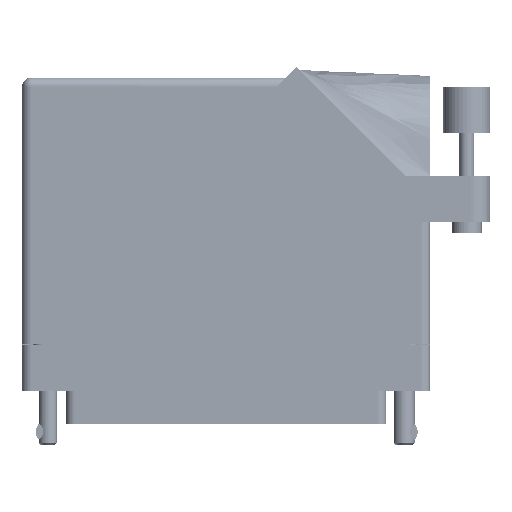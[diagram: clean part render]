
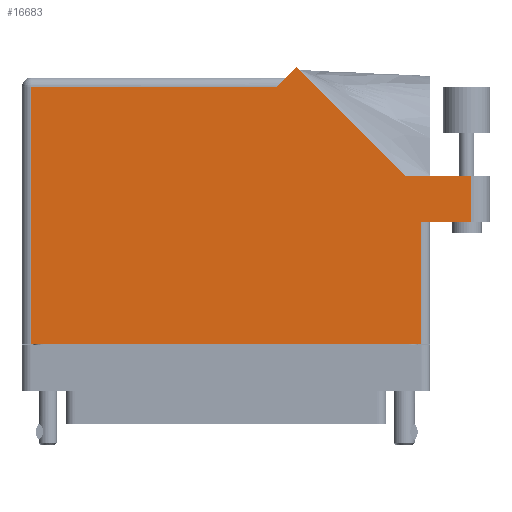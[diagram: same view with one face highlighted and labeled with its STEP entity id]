
A CAD part, front view. The second image highlights one B-rep face of the part: STEP entity #16683.
In plain terms, the highlighted face is planar.
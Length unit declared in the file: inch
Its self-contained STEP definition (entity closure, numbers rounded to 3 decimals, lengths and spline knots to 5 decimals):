
#970 = VERTEX_POINT ( 'NONE', #47959 ) ;
#1449 = CARTESIAN_POINT ( 'NONE',  ( -1.297, -0.1, 0.617 ) ) ;
#1583 = EDGE_CURVE ( 'NONE', #970, #49305, #15791, .T. ) ;
#4131 = VERTEX_POINT ( 'NONE', #48680 ) ;
#9741 = ORIENTED_EDGE ( 'NONE', *, *, #15058, .T. ) ;
#12360 = PLANE ( 'NONE',  #44859 ) ;
#13094 = DIRECTION ( 'NONE',  ( 0., -1., 0. ) ) ;
#14873 = VECTOR ( 'NONE', #26172, 39.37008 ) ;
#15058 = EDGE_CURVE ( 'NONE', #27131, #40115, #57068, .T. ) ;
#15791 = LINE ( 'NONE', #27085, #44267 ) ;
#16536 = LINE ( 'NONE', #63909, #46008 ) ;
#16683 = ADVANCED_FACE ( 'NONE', ( #58656 ), #12360, .F. ) ;
#17166 = VECTOR ( 'NONE', #78746, 39.37008 ) ;
#17698 = VECTOR ( 'NONE', #47633, 39.37008 ) ;
#17883 = ORIENTED_EDGE ( 'NONE', *, *, #66912, .T. ) ;
#19144 = DIRECTION ( 'NONE',  ( -1., 0., 0. ) ) ;
#21097 = CARTESIAN_POINT ( 'NONE',  ( 1.19342, 1.022, 0.617 ) ) ;
#26172 = DIRECTION ( 'NONE',  ( -1., 0., 0. ) ) ;
#26757 = VECTOR ( 'NONE', #80511, 39.37008 ) ;
#27085 = CARTESIAN_POINT ( 'NONE',  ( -1.297, -0.1, 0.617 ) ) ;
#27131 = VERTEX_POINT ( 'NONE', #44527 ) ;
#32243 = CARTESIAN_POINT ( 'NONE',  ( -1.359, 1.675, 0.617 ) ) ;
#34160 = LINE ( 'NONE', #57874, #14873 ) ;
#34805 = ORIENTED_EDGE ( 'NONE', *, *, #36938, .T. ) ;
#35820 = CARTESIAN_POINT ( 'NONE',  ( 1.19342, 1.022, 0.617 ) ) ;
#36662 = ORIENTED_EDGE ( 'NONE', *, *, #62795, .T. ) ;
#36938 = EDGE_CURVE ( 'NONE', #40115, #71398, #34160, .T. ) ;
#37815 = CARTESIAN_POINT ( 'NONE',  ( 1.634, 1.022, 0.617 ) ) ;
#39908 = CARTESIAN_POINT ( 'NONE',  ( 1.297, 0.715, 0.617 ) ) ;
#40115 = VERTEX_POINT ( 'NONE', #64140 ) ;
#44267 = VECTOR ( 'NONE', #13094, 39.37008 ) ;
#44527 = CARTESIAN_POINT ( 'NONE',  ( 1.634, 0.715, 0.617 ) ) ;
#44859 = AXIS2_PLACEMENT_3D ( 'NONE', #32243, #77607, #19144 ) ;
#45929 = VECTOR ( 'NONE', #63627, 39.37008 ) ;
#46008 = VECTOR ( 'NONE', #83530, 39.37008 ) ;
#46422 = ORIENTED_EDGE ( 'NONE', *, *, #1583, .T. ) ;
#47633 = DIRECTION ( 'NONE',  ( -1., 0., 0. ) ) ;
#47959 = CARTESIAN_POINT ( 'NONE',  ( -1.297, 1.613, 0.617 ) ) ;
#48680 = CARTESIAN_POINT ( 'NONE',  ( 1.297, 0.715, 0.617 ) ) ;
#48909 = DIRECTION ( 'NONE',  ( -0.707, 0.707, 0. ) ) ;
#49037 = LINE ( 'NONE', #67720, #26757 ) ;
#49305 = VERTEX_POINT ( 'NONE', #1449 ) ;
#49590 = EDGE_CURVE ( 'NONE', #53070, #970, #69543, .T. ) ;
#52444 = CARTESIAN_POINT ( 'NONE',  ( 1.297, -0.1, 0.617 ) ) ;
#53070 = VERTEX_POINT ( 'NONE', #70966 ) ;
#56089 = ORIENTED_EDGE ( 'NONE', *, *, #71391, .T. ) ;
#56531 = EDGE_CURVE ( 'NONE', #80169, #53070, #49037, .T. ) ;
#56532 = ORIENTED_EDGE ( 'NONE', *, *, #56531, .T. ) ;
#57068 = LINE ( 'NONE', #37815, #45929 ) ;
#57874 = CARTESIAN_POINT ( 'NONE',  ( 1.759, 1.022, 0.617 ) ) ;
#58656 = FACE_OUTER_BOUND ( 'NONE', #78114, .T. ) ;
#59872 = VECTOR ( 'NONE', #78013, 39.37008 ) ;
#60651 = CARTESIAN_POINT ( 'NONE',  ( -1.359, 1.613, 0.617 ) ) ;
#62795 = EDGE_CURVE ( 'NONE', #71398, #80169, #79728, .T. ) ;
#63627 = DIRECTION ( 'NONE',  ( 0., 1., 0. ) ) ;
#63909 = CARTESIAN_POINT ( 'NONE',  ( -1.359, -0.1, 0.617 ) ) ;
#64140 = CARTESIAN_POINT ( 'NONE',  ( 1.634, 1.022, 0.617 ) ) ;
#64615 = VERTEX_POINT ( 'NONE', #52444 ) ;
#65044 = ORIENTED_EDGE ( 'NONE', *, *, #74780, .T. ) ;
#66021 = LINE ( 'NONE', #70649, #59872 ) ;
#66912 = EDGE_CURVE ( 'NONE', #4131, #27131, #66021, .T. ) ;
#67720 = CARTESIAN_POINT ( 'NONE',  ( 0.399, 1.675, 0.617 ) ) ;
#69543 = LINE ( 'NONE', #60651, #17698 ) ;
#70589 = VECTOR ( 'NONE', #48909, 39.37008 ) ;
#70649 = CARTESIAN_POINT ( 'NONE',  ( 1.359, 0.715, 0.617 ) ) ;
#70966 = CARTESIAN_POINT ( 'NONE',  ( 0.337, 1.613, 0.617 ) ) ;
#71024 = LINE ( 'NONE', #39908, #17166 ) ;
#71047 = CARTESIAN_POINT ( 'NONE',  ( 0.46971, 1.74571, 0.617 ) ) ;
#71391 = EDGE_CURVE ( 'NONE', #64615, #4131, #71024, .T. ) ;
#71398 = VERTEX_POINT ( 'NONE', #21097 ) ;
#74780 = EDGE_CURVE ( 'NONE', #49305, #64615, #16536, .T. ) ;
#77607 = DIRECTION ( 'NONE',  ( 0., 0., -1. ) ) ;
#78013 = DIRECTION ( 'NONE',  ( 1., 0., 0. ) ) ;
#78114 = EDGE_LOOP ( 'NONE', ( #17883, #9741, #34805, #36662, #56532, #78344, #46422, #65044, #56089 ) ) ;
#78344 = ORIENTED_EDGE ( 'NONE', *, *, #49590, .T. ) ;
#78746 = DIRECTION ( 'NONE',  ( 0., 1., 0. ) ) ;
#79728 = LINE ( 'NONE', #35820, #70589 ) ;
#80169 = VERTEX_POINT ( 'NONE', #71047 ) ;
#80511 = DIRECTION ( 'NONE',  ( -0.707, -0.707, 0. ) ) ;
#83530 = DIRECTION ( 'NONE',  ( 1., 0., 0. ) ) ;
